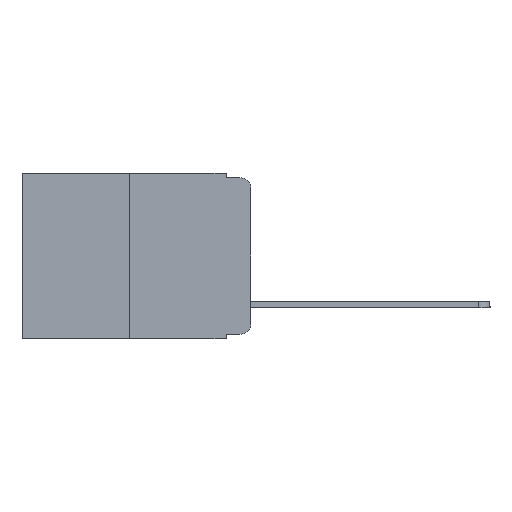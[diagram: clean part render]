
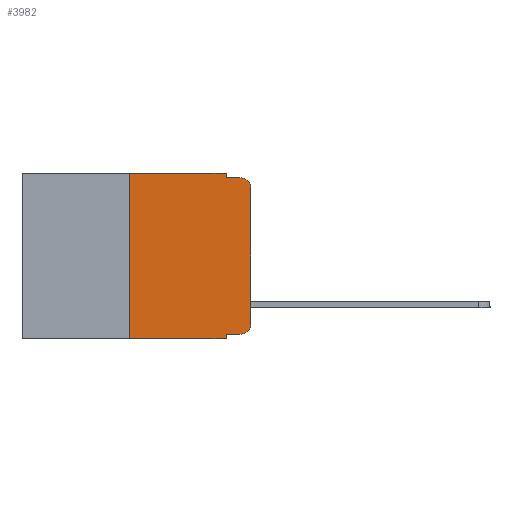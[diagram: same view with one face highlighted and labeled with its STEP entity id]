
A CAD part, left-side view. The second image highlights one B-rep face of the part: STEP entity #3982.
In plain terms, the highlighted planar face has unit normal (-1, 0, 0).
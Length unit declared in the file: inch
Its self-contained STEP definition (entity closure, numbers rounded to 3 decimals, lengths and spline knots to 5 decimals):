
#198 = LINE ( 'NONE', #8148, #7661 ) ;
#456 = CARTESIAN_POINT ( 'NONE',  ( 0., 0.02, -0.03 ) ) ;
#475 = DIRECTION ( 'NONE',  ( 0., 0., -1. ) ) ;
#543 = CIRCLE ( 'NONE', #15364, 0.02 ) ;
#550 = DIRECTION ( 'NONE',  ( 0., 0., -1. ) ) ;
#607 = ORIENTED_EDGE ( 'NONE', *, *, #4331, .F. ) ;
#683 = CARTESIAN_POINT ( 'NONE',  ( 0., 0.02, -0.01 ) ) ;
#1539 = EDGE_CURVE ( 'NONE', #12965, #12530, #11382, .T. ) ;
#1867 = DIRECTION ( 'NONE',  ( -1., 0., 0. ) ) ;
#2415 = ORIENTED_EDGE ( 'NONE', *, *, #2947, .T. ) ;
#2419 = ORIENTED_EDGE ( 'NONE', *, *, #13891, .F. ) ;
#2947 = EDGE_CURVE ( 'NONE', #7867, #6853, #14132, .T. ) ;
#3327 = CARTESIAN_POINT ( 'NONE',  ( 0., 0.051, -0.343 ) ) ;
#3448 = VECTOR ( 'NONE', #17030, 39.37008 ) ;
#3520 = VERTEX_POINT ( 'NONE', #683 ) ;
#3584 = LINE ( 'NONE', #11652, #3448 ) ;
#3904 = DIRECTION ( 'NONE',  ( 0., -1., 0. ) ) ;
#3982 = ADVANCED_FACE ( 'NONE', ( #11332 ), #16700, .F. ) ;
#4039 = VERTEX_POINT ( 'NONE', #14213 ) ;
#4080 = CARTESIAN_POINT ( 'NONE',  ( 0., 0.051, -0.333 ) ) ;
#4090 = CARTESIAN_POINT ( 'NONE',  ( 0., 0.473, -0.343 ) ) ;
#4193 = DIRECTION ( 'NONE',  ( 0., -1., 0. ) ) ;
#4331 = EDGE_CURVE ( 'NONE', #11563, #5613, #8339, .T. ) ;
#4600 = AXIS2_PLACEMENT_3D ( 'NONE', #9917, #1867, #16519 ) ;
#4677 = DIRECTION ( 'NONE',  ( 0., 0., -1. ) ) ;
#5349 = LINE ( 'NONE', #14988, #6247 ) ;
#5613 = VERTEX_POINT ( 'NONE', #3327 ) ;
#5781 = DIRECTION ( 'NONE',  ( 0., 0., -1. ) ) ;
#5889 = ORIENTED_EDGE ( 'NONE', *, *, #13998, .T. ) ;
#5953 = VECTOR ( 'NONE', #12802, 39.37008 ) ;
#5993 = CARTESIAN_POINT ( 'NONE',  ( 0., 0.473, 0. ) ) ;
#6247 = VECTOR ( 'NONE', #16069, 39.37008 ) ;
#6739 = DIRECTION ( 'NONE',  ( -1., 0., 0. ) ) ;
#6853 = VERTEX_POINT ( 'NONE', #15765 ) ;
#6904 = AXIS2_PLACEMENT_3D ( 'NONE', #5993, #7214, #4677 ) ;
#7064 = EDGE_CURVE ( 'NONE', #4039, #12965, #14698, .T. ) ;
#7214 = DIRECTION ( 'NONE',  ( 1., 0., 0. ) ) ;
#7463 = CARTESIAN_POINT ( 'NONE',  ( 0., 0., 0. ) ) ;
#7661 = VECTOR ( 'NONE', #4193, 39.37008 ) ;
#7775 = EDGE_CURVE ( 'NONE', #6853, #3520, #543, .T. ) ;
#7808 = CARTESIAN_POINT ( 'NONE',  ( 0., 0.25, -0.343 ) ) ;
#7867 = VERTEX_POINT ( 'NONE', #12421 ) ;
#7871 = DIRECTION ( 'NONE',  ( 0., -1., 0. ) ) ;
#8148 = CARTESIAN_POINT ( 'NONE',  ( 0., 0.051, -0.333 ) ) ;
#8339 = LINE ( 'NONE', #13863, #8874 ) ;
#8651 = VECTOR ( 'NONE', #550, 39.37008 ) ;
#8874 = VECTOR ( 'NONE', #475, 39.37008 ) ;
#8925 = ORIENTED_EDGE ( 'NONE', *, *, #16242, .T. ) ;
#9526 = LINE ( 'NONE', #4090, #11294 ) ;
#9917 = CARTESIAN_POINT ( 'NONE',  ( 0., 0.02, -0.313 ) ) ;
#11294 = VECTOR ( 'NONE', #7871, 39.37008 ) ;
#11332 = FACE_OUTER_BOUND ( 'NONE', #11569, .T. ) ;
#11341 = ORIENTED_EDGE ( 'NONE', *, *, #1539, .F. ) ;
#11382 = LINE ( 'NONE', #16753, #8651 ) ;
#11563 = VERTEX_POINT ( 'NONE', #4080 ) ;
#11569 = EDGE_LOOP ( 'NONE', ( #2415, #14045, #14970, #11341, #11888, #2419, #8925, #607, #5889, #12313 ) ) ;
#11652 = CARTESIAN_POINT ( 'NONE',  ( 0., 0.25, 0. ) ) ;
#11888 = ORIENTED_EDGE ( 'NONE', *, *, #7064, .F. ) ;
#12142 = CIRCLE ( 'NONE', #4600, 0.02 ) ;
#12313 = ORIENTED_EDGE ( 'NONE', *, *, #14290, .T. ) ;
#12421 = CARTESIAN_POINT ( 'NONE',  ( 0., 0., -0.313 ) ) ;
#12530 = VERTEX_POINT ( 'NONE', #14258 ) ;
#12802 = DIRECTION ( 'NONE',  ( 0., 0., 1. ) ) ;
#12965 = VERTEX_POINT ( 'NONE', #15486 ) ;
#13279 = CARTESIAN_POINT ( 'NONE',  ( 0., 0.473, 0. ) ) ;
#13437 = VERTEX_POINT ( 'NONE', #14568 ) ;
#13863 = CARTESIAN_POINT ( 'NONE',  ( 0., 0.051, 0. ) ) ;
#13891 = EDGE_CURVE ( 'NONE', #14491, #4039, #3584, .T. ) ;
#13998 = EDGE_CURVE ( 'NONE', #11563, #13437, #198, .T. ) ;
#14045 = ORIENTED_EDGE ( 'NONE', *, *, #7775, .T. ) ;
#14132 = LINE ( 'NONE', #7463, #5953 ) ;
#14213 = CARTESIAN_POINT ( 'NONE',  ( 0., 0.25, 0. ) ) ;
#14258 = CARTESIAN_POINT ( 'NONE',  ( 0., 0.051, -0.01 ) ) ;
#14290 = EDGE_CURVE ( 'NONE', #13437, #7867, #12142, .T. ) ;
#14491 = VERTEX_POINT ( 'NONE', #7808 ) ;
#14507 = VECTOR ( 'NONE', #3904, 39.37008 ) ;
#14568 = CARTESIAN_POINT ( 'NONE',  ( 0., 0.02, -0.333 ) ) ;
#14698 = LINE ( 'NONE', #13279, #14507 ) ;
#14970 = ORIENTED_EDGE ( 'NONE', *, *, #17203, .F. ) ;
#14988 = CARTESIAN_POINT ( 'NONE',  ( 0., 0.051, -0.01 ) ) ;
#15364 = AXIS2_PLACEMENT_3D ( 'NONE', #456, #6739, #5781 ) ;
#15486 = CARTESIAN_POINT ( 'NONE',  ( 0., 0.051, 0. ) ) ;
#15765 = CARTESIAN_POINT ( 'NONE',  ( 0., 0., -0.03 ) ) ;
#16069 = DIRECTION ( 'NONE',  ( 0., -1., 0. ) ) ;
#16242 = EDGE_CURVE ( 'NONE', #14491, #5613, #9526, .T. ) ;
#16519 = DIRECTION ( 'NONE',  ( 0., 0., -1. ) ) ;
#16700 = PLANE ( 'NONE',  #6904 ) ;
#16753 = CARTESIAN_POINT ( 'NONE',  ( 0., 0.051, 0. ) ) ;
#17030 = DIRECTION ( 'NONE',  ( 0., 0., 1. ) ) ;
#17203 = EDGE_CURVE ( 'NONE', #12530, #3520, #5349, .T. ) ;
